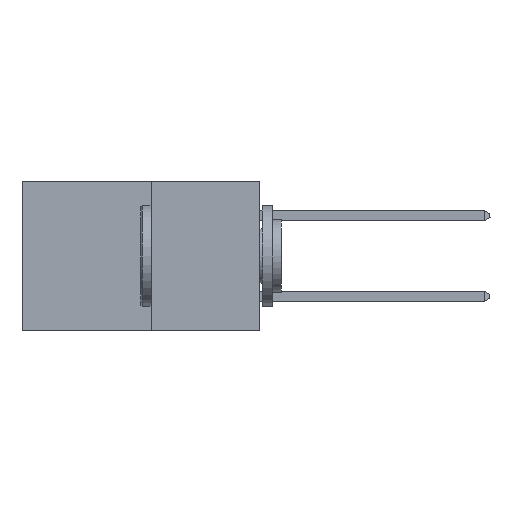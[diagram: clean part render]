
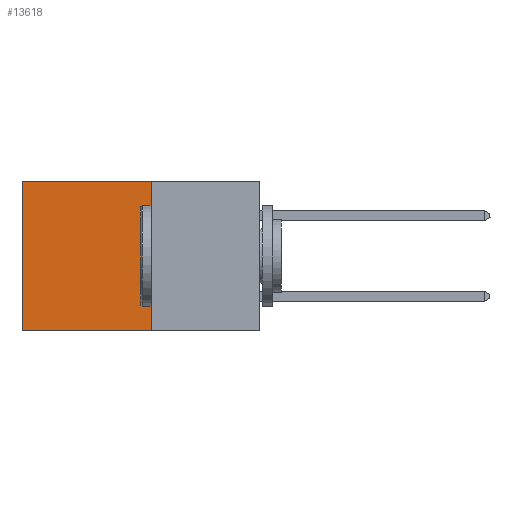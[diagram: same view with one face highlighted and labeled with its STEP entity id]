
A CAD part, left-side view. The second image highlights one B-rep face of the part: STEP entity #13618.
In plain terms, the highlighted planar face has unit normal (-1, 0, 0).
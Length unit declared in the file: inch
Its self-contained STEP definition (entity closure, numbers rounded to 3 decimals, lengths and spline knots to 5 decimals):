
#159 = DIRECTION ( 'NONE',  ( 1., 0., 0. ) ) ;
#488 = CARTESIAN_POINT ( 'NONE',  ( 0.277, 0.27, -0.37 ) ) ;
#1516 = VECTOR ( 'NONE', #18637, 39.37008 ) ;
#1843 = CARTESIAN_POINT ( 'NONE',  ( 0.277, 0.27, -0.37 ) ) ;
#2004 = VECTOR ( 'NONE', #16981, 39.37008 ) ;
#4421 = DIRECTION ( 'NONE',  ( 0., 0., -1. ) ) ;
#6010 = CARTESIAN_POINT ( 'NONE',  ( 0.277, 0.59, 0. ) ) ;
#6503 = CARTESIAN_POINT ( 'NONE',  ( 0.277, 0.27, 0. ) ) ;
#6597 = EDGE_CURVE ( 'NONE', #26143, #20726, #12901, .T. ) ;
#7853 = PLANE ( 'NONE',  #18337 ) ;
#8077 = FACE_OUTER_BOUND ( 'NONE', #15669, .T. ) ;
#8327 = CARTESIAN_POINT ( 'NONE',  ( 0.277, 0.59, -0.37 ) ) ;
#8375 = LINE ( 'NONE', #488, #1516 ) ;
#8456 = ORIENTED_EDGE ( 'NONE', *, *, #29888, .T. ) ;
#8782 = DIRECTION ( 'NONE',  ( 0., 0., -1. ) ) ;
#9407 = CARTESIAN_POINT ( 'NONE',  ( 0.277, 0.27, 0. ) ) ;
#9975 = ORIENTED_EDGE ( 'NONE', *, *, #31003, .F. ) ;
#10326 = ORIENTED_EDGE ( 'NONE', *, *, #15146, .F. ) ;
#11205 = VERTEX_POINT ( 'NONE', #9407 ) ;
#11776 = CARTESIAN_POINT ( 'NONE',  ( 0.277, 0.27, -0.37 ) ) ;
#12901 = LINE ( 'NONE', #8327, #25733 ) ;
#13101 = CARTESIAN_POINT ( 'NONE',  ( 0.277, 0.27, -0.37 ) ) ;
#13618 = ADVANCED_FACE ( 'NONE', ( #8077 ), #7853, .F. ) ;
#15146 = EDGE_CURVE ( 'NONE', #11205, #23647, #19026, .T. ) ;
#15669 = EDGE_LOOP ( 'NONE', ( #23195, #9975, #10326, #8456 ) ) ;
#15835 = LINE ( 'NONE', #6503, #2004 ) ;
#16981 = DIRECTION ( 'NONE',  ( 0., 1., 0. ) ) ;
#17651 = CARTESIAN_POINT ( 'NONE',  ( 0.277, 0.59, -0.37 ) ) ;
#18327 = DIRECTION ( 'NONE',  ( 0., 0., -1. ) ) ;
#18337 = AXIS2_PLACEMENT_3D ( 'NONE', #13101, #159, #18327 ) ;
#18637 = DIRECTION ( 'NONE',  ( 0., 1., 0. ) ) ;
#19026 = LINE ( 'NONE', #1843, #31702 ) ;
#20726 = VERTEX_POINT ( 'NONE', #17651 ) ;
#23195 = ORIENTED_EDGE ( 'NONE', *, *, #6597, .T. ) ;
#23647 = VERTEX_POINT ( 'NONE', #11776 ) ;
#25733 = VECTOR ( 'NONE', #8782, 39.37008 ) ;
#26143 = VERTEX_POINT ( 'NONE', #6010 ) ;
#29888 = EDGE_CURVE ( 'NONE', #11205, #26143, #15835, .T. ) ;
#31003 = EDGE_CURVE ( 'NONE', #23647, #20726, #8375, .T. ) ;
#31702 = VECTOR ( 'NONE', #4421, 39.37008 ) ;
